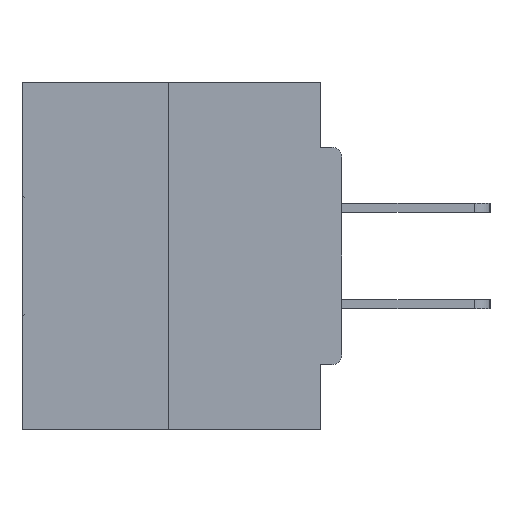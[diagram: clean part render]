
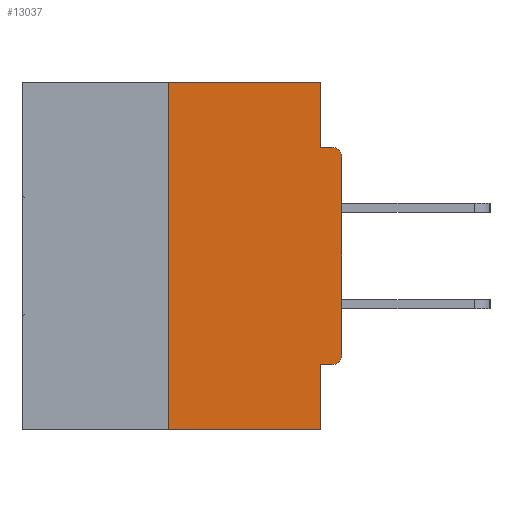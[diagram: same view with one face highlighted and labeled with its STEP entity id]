
A CAD part, left-side view. The second image highlights one B-rep face of the part: STEP entity #13037.
In plain terms, the highlighted planar face has unit normal (-1, 0, 0).
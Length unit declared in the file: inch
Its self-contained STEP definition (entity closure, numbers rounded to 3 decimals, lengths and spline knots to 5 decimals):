
#290 = CARTESIAN_POINT ( 'NONE',  ( 0., 0.46, 0. ) ) ;
#489 = EDGE_CURVE ( 'NONE', #18566, #8091, #37811, .T. ) ;
#1274 = ORIENTED_EDGE ( 'NONE', *, *, #15832, .T. ) ;
#2878 = LINE ( 'NONE', #18866, #11976 ) ;
#3062 = CARTESIAN_POINT ( 'NONE',  ( 0., 0.031, 0. ) ) ;
#3669 = AXIS2_PLACEMENT_3D ( 'NONE', #22385, #4082, #7171 ) ;
#4082 = DIRECTION ( 'NONE',  ( -1., 0., 0. ) ) ;
#5747 = CARTESIAN_POINT ( 'NONE',  ( 0., 0.25, 0. ) ) ;
#6240 = DIRECTION ( 'NONE',  ( 0., -1., 0. ) ) ;
#6290 = DIRECTION ( 'NONE',  ( 0., 0., -1. ) ) ;
#6351 = CARTESIAN_POINT ( 'NONE',  ( 0., 0., -0.3915 ) ) ;
#6566 = LINE ( 'NONE', #9177, #32356 ) ;
#7164 = CARTESIAN_POINT ( 'NONE',  ( 0., 0.015, -0.1085 ) ) ;
#7171 = DIRECTION ( 'NONE',  ( 0., 0., -1. ) ) ;
#7893 = EDGE_CURVE ( 'NONE', #10061, #26963, #19166, .T. ) ;
#8091 = VERTEX_POINT ( 'NONE', #24534 ) ;
#9024 = AXIS2_PLACEMENT_3D ( 'NONE', #7164, #34144, #18929 ) ;
#9177 = CARTESIAN_POINT ( 'NONE',  ( 0., 0.46, -0.5 ) ) ;
#10061 = VERTEX_POINT ( 'NONE', #29017 ) ;
#10378 = EDGE_CURVE ( 'NONE', #20599, #11016, #11264, .T. ) ;
#10771 = LINE ( 'NONE', #3062, #34180 ) ;
#10904 = CARTESIAN_POINT ( 'NONE',  ( 0., 0., -0.4065 ) ) ;
#10978 = VERTEX_POINT ( 'NONE', #6351 ) ;
#11016 = VERTEX_POINT ( 'NONE', #27211 ) ;
#11252 = CARTESIAN_POINT ( 'NONE',  ( 0., 0.031, -0.5 ) ) ;
#11264 = LINE ( 'NONE', #18286, #26603 ) ;
#11632 = CARTESIAN_POINT ( 'NONE',  ( 0., 0., 0. ) ) ;
#11976 = VECTOR ( 'NONE', #30894, 39.37008 ) ;
#12459 = CARTESIAN_POINT ( 'NONE',  ( 0., 0.031, -0.4065 ) ) ;
#12892 = ORIENTED_EDGE ( 'NONE', *, *, #30370, .F. ) ;
#13037 = ADVANCED_FACE ( 'NONE', ( #25998 ), #36894, .F. ) ;
#15701 = VECTOR ( 'NONE', #21140, 39.37008 ) ;
#15832 = EDGE_CURVE ( 'NONE', #25686, #8091, #24300, .T. ) ;
#17827 = EDGE_CURVE ( 'NONE', #10061, #10978, #18797, .T. ) ;
#18286 = CARTESIAN_POINT ( 'NONE',  ( 0., 0.46, 0. ) ) ;
#18566 = VERTEX_POINT ( 'NONE', #22727 ) ;
#18797 = CIRCLE ( 'NONE', #3669, 0.015 ) ;
#18866 = CARTESIAN_POINT ( 'NONE',  ( 0., 0.031, -0.5 ) ) ;
#18929 = DIRECTION ( 'NONE',  ( 0., 0., -1. ) ) ;
#19166 = LINE ( 'NONE', #10904, #19625 ) ;
#19559 = LINE ( 'NONE', #20759, #15701 ) ;
#19625 = VECTOR ( 'NONE', #35620, 39.37008 ) ;
#20599 = VERTEX_POINT ( 'NONE', #5747 ) ;
#20759 = CARTESIAN_POINT ( 'NONE',  ( 0., 0.25, 0. ) ) ;
#20878 = ORIENTED_EDGE ( 'NONE', *, *, #10378, .F. ) ;
#21140 = DIRECTION ( 'NONE',  ( 0., 0., 1. ) ) ;
#21309 = EDGE_CURVE ( 'NONE', #26963, #33253, #2878, .T. ) ;
#21395 = DIRECTION ( 'NONE',  ( 1., 0., 0. ) ) ;
#21664 = ORIENTED_EDGE ( 'NONE', *, *, #37944, .F. ) ;
#22385 = CARTESIAN_POINT ( 'NONE',  ( 0., 0.015, -0.3915 ) ) ;
#22559 = ORIENTED_EDGE ( 'NONE', *, *, #489, .F. ) ;
#22727 = CARTESIAN_POINT ( 'NONE',  ( 0., 0.031, -0.0935 ) ) ;
#22771 = AXIS2_PLACEMENT_3D ( 'NONE', #290, #21395, #30514 ) ;
#23464 = ORIENTED_EDGE ( 'NONE', *, *, #7893, .F. ) ;
#24300 = CIRCLE ( 'NONE', #9024, 0.015 ) ;
#24534 = CARTESIAN_POINT ( 'NONE',  ( 0., 0.015, -0.0935 ) ) ;
#25686 = VERTEX_POINT ( 'NONE', #30597 ) ;
#25998 = FACE_OUTER_BOUND ( 'NONE', #35253, .T. ) ;
#26603 = VECTOR ( 'NONE', #30329, 39.37008 ) ;
#26963 = VERTEX_POINT ( 'NONE', #12459 ) ;
#26965 = ORIENTED_EDGE ( 'NONE', *, *, #17827, .T. ) ;
#27211 = CARTESIAN_POINT ( 'NONE',  ( 0., 0.031, 0. ) ) ;
#28773 = VECTOR ( 'NONE', #33117, 39.37008 ) ;
#29017 = CARTESIAN_POINT ( 'NONE',  ( 0., 0.015, -0.4065 ) ) ;
#29632 = LINE ( 'NONE', #11632, #36750 ) ;
#30329 = DIRECTION ( 'NONE',  ( 0., -1., 0. ) ) ;
#30370 = EDGE_CURVE ( 'NONE', #11016, #18566, #10771, .T. ) ;
#30514 = DIRECTION ( 'NONE',  ( 0., 0., -1. ) ) ;
#30597 = CARTESIAN_POINT ( 'NONE',  ( 0., 0., -0.1085 ) ) ;
#30894 = DIRECTION ( 'NONE',  ( 0., 0., -1. ) ) ;
#32356 = VECTOR ( 'NONE', #6240, 39.37008 ) ;
#33117 = DIRECTION ( 'NONE',  ( 0., -1., 0. ) ) ;
#33253 = VERTEX_POINT ( 'NONE', #11252 ) ;
#33888 = VERTEX_POINT ( 'NONE', #38920 ) ;
#34144 = DIRECTION ( 'NONE',  ( -1., 0., 0. ) ) ;
#34180 = VECTOR ( 'NONE', #6290, 39.37008 ) ;
#34417 = EDGE_CURVE ( 'NONE', #10978, #25686, #29632, .T. ) ;
#35214 = EDGE_CURVE ( 'NONE', #33888, #33253, #6566, .T. ) ;
#35253 = EDGE_LOOP ( 'NONE', ( #20878, #21664, #38510, #38395, #23464, #26965, #37146, #1274, #22559, #12892 ) ) ;
#35620 = DIRECTION ( 'NONE',  ( 0., 1., 0. ) ) ;
#36750 = VECTOR ( 'NONE', #39149, 39.37008 ) ;
#36894 = PLANE ( 'NONE',  #22771 ) ;
#37146 = ORIENTED_EDGE ( 'NONE', *, *, #34417, .T. ) ;
#37811 = LINE ( 'NONE', #39403, #28773 ) ;
#37944 = EDGE_CURVE ( 'NONE', #33888, #20599, #19559, .T. ) ;
#38395 = ORIENTED_EDGE ( 'NONE', *, *, #21309, .F. ) ;
#38510 = ORIENTED_EDGE ( 'NONE', *, *, #35214, .T. ) ;
#38920 = CARTESIAN_POINT ( 'NONE',  ( 0., 0.25, -0.5 ) ) ;
#39149 = DIRECTION ( 'NONE',  ( 0., 0., 1. ) ) ;
#39403 = CARTESIAN_POINT ( 'NONE',  ( 0., 0., -0.0935 ) ) ;
